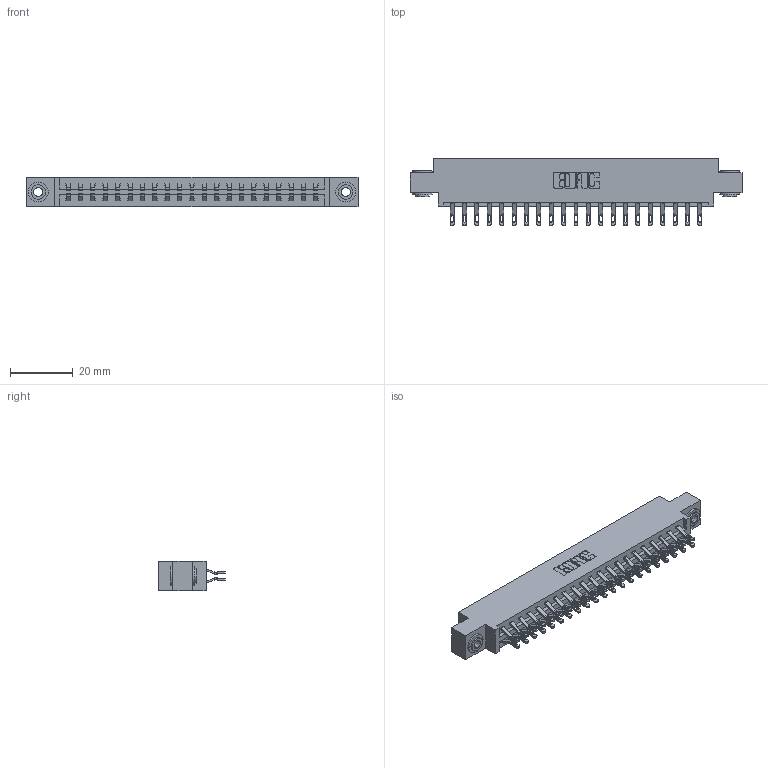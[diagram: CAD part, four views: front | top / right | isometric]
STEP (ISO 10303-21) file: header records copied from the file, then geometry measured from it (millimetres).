
FILE_DESCRIPTION (( 'STEP AP203' ), '1' );
FILE_NAME ('337-042-555-803.STEP', '2019-10-11T13:00:35', ( '' ), ( '' ), 'SwSTEP 2.0', 'SolidWorks 2016', '' );
FILE_SCHEMA (( 'CONFIG_CONTROL_DESIGN' ));
Length unit declared in the file: inch
Products named in the file (4): 345-250-002_345-250-002-102; 337 Part_0.170 Offset - 0.156 Dia-TH; 345-292-001_555 Tail; 337-042-555-803
Assembly tree (45 placements, depth 2):
  337-042-555-803
    337 Part_0.170 Offset - 0.156 Dia-TH
    345-292-001_555 Tail  x42
    345-250-002_345-250-002-102  x2
Bounding box: 106.22 x 21.47 x 9.4 mm (x, y, z)
Volume: 10938.8 mm3; surface area: 12953.7 mm2
Topology: 45 solids, 45 shells, 2676 faces, 8337 edges, 5554 vertices
Faces by surface type: plane 1596, cylinder 1072, cone 8
Entity records: 20106 total; most frequent: CARTESIAN_POINT 3415, ORIENTED_EDGE 3314, DIRECTION 2947, EDGE_CURVE 1657, VECTOR 1485, LINE 1485, VERTEX_POINT 1102, AXIS2_PLACEMENT_3D 731
